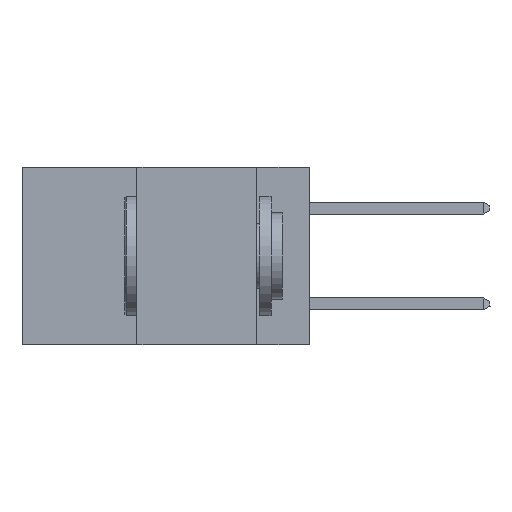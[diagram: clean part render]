
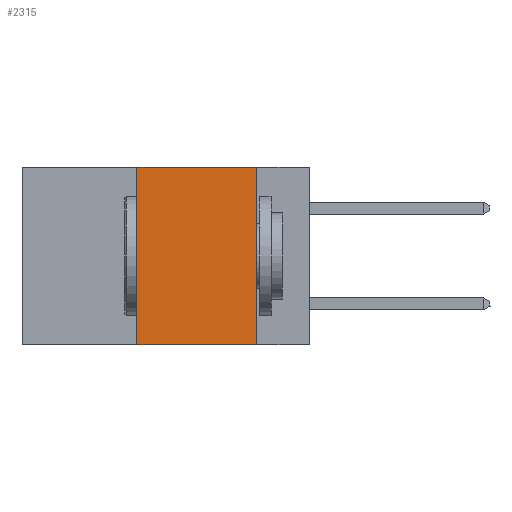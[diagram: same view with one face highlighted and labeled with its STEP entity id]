
A CAD part, left-side view. The second image highlights one B-rep face of the part: STEP entity #2315.
In plain terms, the highlighted planar face has unit normal (-1, 0, 0).
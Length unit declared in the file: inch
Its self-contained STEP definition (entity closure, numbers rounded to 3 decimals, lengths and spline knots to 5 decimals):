
#1789 = CARTESIAN_POINT ( 'NONE',  ( 0., 0.36, 0. ) ) ;
#2315 = ADVANCED_FACE ( 'NONE', ( #3262 ), #4576, .F. ) ;
#3262 = FACE_OUTER_BOUND ( 'NONE', #9733, .T. ) ;
#3968 = VERTEX_POINT ( 'NONE', #1789 ) ;
#4332 = VERTEX_POINT ( 'NONE', #20886 ) ;
#4576 = PLANE ( 'NONE',  #12704 ) ;
#5581 = LINE ( 'NONE', #9975, #16101 ) ;
#5686 = ORIENTED_EDGE ( 'NONE', *, *, #6391, .F. ) ;
#6391 = EDGE_CURVE ( 'NONE', #3968, #4332, #21155, .T. ) ;
#6644 = VECTOR ( 'NONE', #17691, 39.37008 ) ;
#8951 = CARTESIAN_POINT ( 'NONE',  ( 0., 0.36, -0.37 ) ) ;
#9733 = EDGE_LOOP ( 'NONE', ( #20577, #5686, #12950, #20955 ) ) ;
#9975 = CARTESIAN_POINT ( 'NONE',  ( 0., 0.36, 0. ) ) ;
#10182 = DIRECTION ( 'NONE',  ( 0., -1., 0. ) ) ;
#10630 = CARTESIAN_POINT ( 'NONE',  ( 0., 0.6, -0.37 ) ) ;
#11367 = LINE ( 'NONE', #18275, #14468 ) ;
#11628 = EDGE_CURVE ( 'NONE', #4332, #12265, #11367, .T. ) ;
#12265 = VERTEX_POINT ( 'NONE', #13250 ) ;
#12704 = AXIS2_PLACEMENT_3D ( 'NONE', #17493, #17344, #19265 ) ;
#12950 = ORIENTED_EDGE ( 'NONE', *, *, #14585, .F. ) ;
#12982 = DIRECTION ( 'NONE',  ( 0., 0., -1. ) ) ;
#13250 = CARTESIAN_POINT ( 'NONE',  ( 0., 0.11, -0.37 ) ) ;
#14468 = VECTOR ( 'NONE', #12982, 39.37008 ) ;
#14585 = EDGE_CURVE ( 'NONE', #22476, #3968, #5581, .T. ) ;
#14670 = VECTOR ( 'NONE', #10182, 39.37008 ) ;
#16078 = EDGE_CURVE ( 'NONE', #22476, #12265, #22194, .T. ) ;
#16101 = VECTOR ( 'NONE', #20801, 39.37008 ) ;
#16623 = CARTESIAN_POINT ( 'NONE',  ( 0., 0.6, 0. ) ) ;
#17344 = DIRECTION ( 'NONE',  ( 1., 0., 0. ) ) ;
#17493 = CARTESIAN_POINT ( 'NONE',  ( 0., 0.6, 0. ) ) ;
#17691 = DIRECTION ( 'NONE',  ( 0., -1., 0. ) ) ;
#18275 = CARTESIAN_POINT ( 'NONE',  ( 0., 0.11, 0. ) ) ;
#19265 = DIRECTION ( 'NONE',  ( 0., 0., -1. ) ) ;
#20577 = ORIENTED_EDGE ( 'NONE', *, *, #11628, .F. ) ;
#20801 = DIRECTION ( 'NONE',  ( 0., 0., 1. ) ) ;
#20886 = CARTESIAN_POINT ( 'NONE',  ( 0., 0.11, 0. ) ) ;
#20955 = ORIENTED_EDGE ( 'NONE', *, *, #16078, .T. ) ;
#21155 = LINE ( 'NONE', #16623, #14670 ) ;
#22194 = LINE ( 'NONE', #10630, #6644 ) ;
#22476 = VERTEX_POINT ( 'NONE', #8951 ) ;
